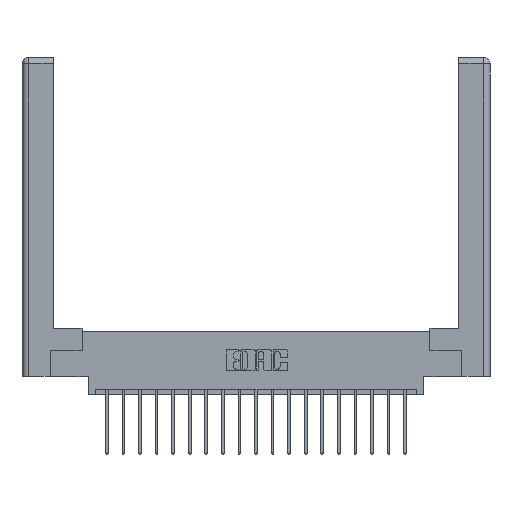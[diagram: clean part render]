
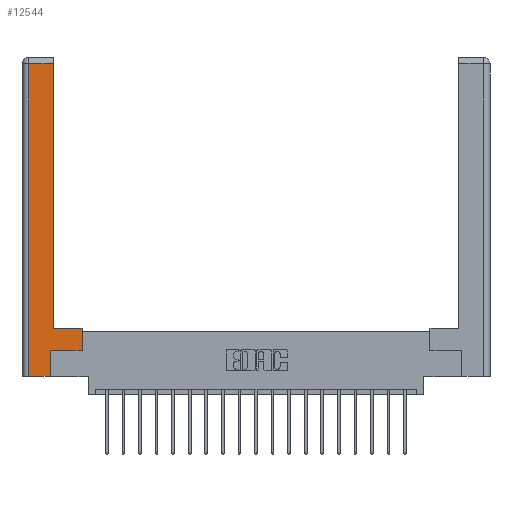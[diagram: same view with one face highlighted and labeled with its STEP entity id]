
A CAD part, top view. The second image highlights one B-rep face of the part: STEP entity #12544.
In plain terms, the highlighted planar face has unit normal (0, 0, 1).
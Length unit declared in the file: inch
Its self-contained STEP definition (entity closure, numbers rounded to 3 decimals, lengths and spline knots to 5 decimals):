
#82 = EDGE_CURVE ( 'NONE', #13319, #10410, #3213, .T. ) ;
#575 = EDGE_CURVE ( 'NONE', #19642, #11375, #20045, .T. ) ;
#1286 = CARTESIAN_POINT ( 'NONE',  ( 0.295, 0.45, 0. ) ) ;
#1570 = ORIENTED_EDGE ( 'NONE', *, *, #6636, .T. ) ;
#1717 = CARTESIAN_POINT ( 'NONE',  ( 0.295, 0.45, 0. ) ) ;
#1914 = ORIENTED_EDGE ( 'NONE', *, *, #6886, .T. ) ;
#2209 = CARTESIAN_POINT ( 'NONE',  ( 0.565, 0.245, 0. ) ) ;
#2478 = CARTESIAN_POINT ( 'NONE',  ( 0.0615, 2.94, 0. ) ) ;
#2605 = CARTESIAN_POINT ( 'NONE',  ( 0.295, 2.94, 0. ) ) ;
#2640 = DIRECTION ( 'NONE',  ( -1., 0., 0. ) ) ;
#2774 = CARTESIAN_POINT ( 'NONE',  ( 0., 0., 0. ) ) ;
#2946 = LINE ( 'NONE', #4673, #17805 ) ;
#3213 = LINE ( 'NONE', #2478, #12665 ) ;
#3508 = FACE_OUTER_BOUND ( 'NONE', #8481, .T. ) ;
#4486 = DIRECTION ( 'NONE',  ( 0., 1., 0. ) ) ;
#4673 = CARTESIAN_POINT ( 'NONE',  ( 0.0615, 0., 0. ) ) ;
#5530 = CARTESIAN_POINT ( 'NONE',  ( 0.565, 0.45, 0. ) ) ;
#5658 = VERTEX_POINT ( 'NONE', #19323 ) ;
#5763 = VECTOR ( 'NONE', #4486, 39.37008 ) ;
#5910 = VECTOR ( 'NONE', #16329, 39.37008 ) ;
#5962 = CARTESIAN_POINT ( 'NONE',  ( 0.265, 0.245, 0. ) ) ;
#6063 = DIRECTION ( 'NONE',  ( -1., 0., 0. ) ) ;
#6636 = EDGE_CURVE ( 'NONE', #10410, #5658, #2946, .T. ) ;
#6886 = EDGE_CURVE ( 'NONE', #9210, #19642, #12103, .T. ) ;
#7195 = DIRECTION ( 'NONE',  ( -1., 0., 0. ) ) ;
#7481 = LINE ( 'NONE', #15336, #5763 ) ;
#7630 = ORIENTED_EDGE ( 'NONE', *, *, #19194, .T. ) ;
#7954 = CARTESIAN_POINT ( 'NONE',  ( 0.565, 0.45, 0. ) ) ;
#8117 = CARTESIAN_POINT ( 'NONE',  ( 0.265, 0., 0. ) ) ;
#8198 = DIRECTION ( 'NONE',  ( 1., 0., 0. ) ) ;
#8302 = ORIENTED_EDGE ( 'NONE', *, *, #575, .T. ) ;
#8481 = EDGE_LOOP ( 'NONE', ( #15080, #13729, #1570, #7630, #14710, #11734, #1914, #8302 ) ) ;
#8838 = DIRECTION ( 'NONE',  ( 0., 1., 0. ) ) ;
#9210 = VERTEX_POINT ( 'NONE', #11092 ) ;
#10138 = LINE ( 'NONE', #2209, #5910 ) ;
#10410 = VERTEX_POINT ( 'NONE', #13809 ) ;
#10748 = DIRECTION ( 'NONE',  ( 0., 0., -1. ) ) ;
#11092 = CARTESIAN_POINT ( 'NONE',  ( 0.565, 0.245, 0. ) ) ;
#11375 = VERTEX_POINT ( 'NONE', #1717 ) ;
#11734 = ORIENTED_EDGE ( 'NONE', *, *, #16928, .T. ) ;
#12103 = LINE ( 'NONE', #5530, #16549 ) ;
#12105 = CARTESIAN_POINT ( 'NONE',  ( 0.265, 0., 0. ) ) ;
#12451 = AXIS2_PLACEMENT_3D ( 'NONE', #2774, #10748, #2640 ) ;
#12544 = ADVANCED_FACE ( 'NONE', ( #3508 ), #15419, .F. ) ;
#12665 = VECTOR ( 'NONE', #7195, 39.37008 ) ;
#12902 = LINE ( 'NONE', #5962, #17040 ) ;
#13295 = CARTESIAN_POINT ( 'NONE',  ( 0.265, 0.245, 0. ) ) ;
#13319 = VERTEX_POINT ( 'NONE', #2605 ) ;
#13695 = EDGE_CURVE ( 'NONE', #19957, #16908, #12902, .T. ) ;
#13729 = ORIENTED_EDGE ( 'NONE', *, *, #82, .T. ) ;
#13809 = CARTESIAN_POINT ( 'NONE',  ( 0.0615, 2.94, 0. ) ) ;
#13845 = DIRECTION ( 'NONE',  ( 0., 1., 0. ) ) ;
#14710 = ORIENTED_EDGE ( 'NONE', *, *, #13695, .T. ) ;
#15080 = ORIENTED_EDGE ( 'NONE', *, *, #20241, .T. ) ;
#15336 = CARTESIAN_POINT ( 'NONE',  ( 0.295, 3., 0. ) ) ;
#15419 = PLANE ( 'NONE',  #12451 ) ;
#15950 = VECTOR ( 'NONE', #8198, 39.37008 ) ;
#16329 = DIRECTION ( 'NONE',  ( 1., 0., 0. ) ) ;
#16549 = VECTOR ( 'NONE', #8838, 39.37008 ) ;
#16908 = VERTEX_POINT ( 'NONE', #13295 ) ;
#16928 = EDGE_CURVE ( 'NONE', #16908, #9210, #10138, .T. ) ;
#17040 = VECTOR ( 'NONE', #13845, 39.37008 ) ;
#17168 = DIRECTION ( 'NONE',  ( 0., -1., 0. ) ) ;
#17287 = VECTOR ( 'NONE', #6063, 39.37008 ) ;
#17805 = VECTOR ( 'NONE', #17168, 39.37008 ) ;
#19194 = EDGE_CURVE ( 'NONE', #5658, #19957, #20202, .T. ) ;
#19323 = CARTESIAN_POINT ( 'NONE',  ( 0.0615, 0., 0. ) ) ;
#19642 = VERTEX_POINT ( 'NONE', #7954 ) ;
#19957 = VERTEX_POINT ( 'NONE', #12105 ) ;
#20045 = LINE ( 'NONE', #1286, #17287 ) ;
#20202 = LINE ( 'NONE', #8117, #15950 ) ;
#20241 = EDGE_CURVE ( 'NONE', #11375, #13319, #7481, .T. ) ;
